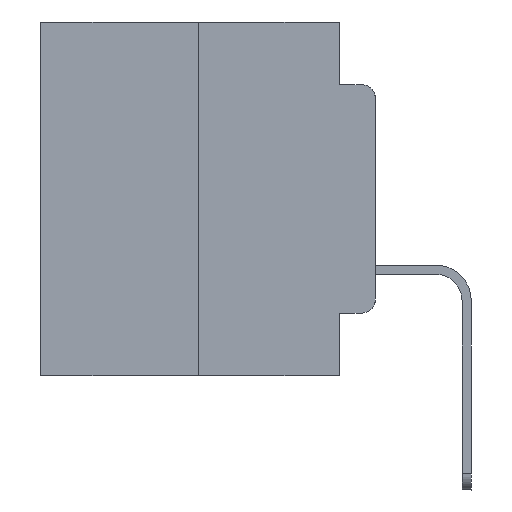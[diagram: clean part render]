
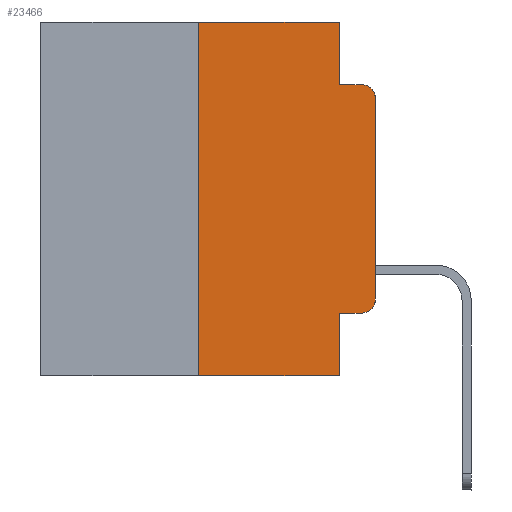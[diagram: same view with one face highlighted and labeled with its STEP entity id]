
A CAD part, left-side view. The second image highlights one B-rep face of the part: STEP entity #23466.
In plain terms, the highlighted planar face has unit normal (-1, 0, 0).
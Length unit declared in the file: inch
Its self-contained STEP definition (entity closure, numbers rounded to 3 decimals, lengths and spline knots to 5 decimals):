
#90 = EDGE_LOOP ( 'NONE', ( #7906, #20675, #12729, #15531, #20696, #12581, #9927, #1979, #15007, #8312 ) ) ;
#669 = VECTOR ( 'NONE', #8764, 39.37008 ) ;
#804 = LINE ( 'NONE', #24019, #14178 ) ;
#986 = LINE ( 'NONE', #20021, #14971 ) ;
#1452 = EDGE_CURVE ( 'NONE', #23525, #15380, #804, .T. ) ;
#1881 = LINE ( 'NONE', #20038, #669 ) ;
#1979 = ORIENTED_EDGE ( 'NONE', *, *, #7526, .F. ) ;
#1997 = VERTEX_POINT ( 'NONE', #24059 ) ;
#2972 = CARTESIAN_POINT ( 'NONE',  ( 0., 0., -0.3915 ) ) ;
#3052 = CARTESIAN_POINT ( 'NONE',  ( 0., 0.473, 0. ) ) ;
#3408 = FACE_OUTER_BOUND ( 'NONE', #90, .T. ) ;
#3547 = VECTOR ( 'NONE', #22465, 39.37008 ) ;
#4702 = DIRECTION ( 'NONE',  ( 0., -1., 0. ) ) ;
#4717 = EDGE_CURVE ( 'NONE', #17170, #5375, #19587, .T. ) ;
#4892 = LINE ( 'NONE', #21923, #9534 ) ;
#5129 = VERTEX_POINT ( 'NONE', #7682 ) ;
#5156 = DIRECTION ( 'NONE',  ( -1., 0., 0. ) ) ;
#5375 = VERTEX_POINT ( 'NONE', #7181 ) ;
#5620 = EDGE_CURVE ( 'NONE', #17170, #1997, #10167, .T. ) ;
#6285 = EDGE_CURVE ( 'NONE', #5375, #25774, #11062, .T. ) ;
#6389 = CARTESIAN_POINT ( 'NONE',  ( 0., 0.25, -0.5 ) ) ;
#7024 = VECTOR ( 'NONE', #4702, 39.37008 ) ;
#7181 = CARTESIAN_POINT ( 'NONE',  ( 0., 0.25, 0. ) ) ;
#7294 = CARTESIAN_POINT ( 'NONE',  ( 0., 0.02, -0.1085 ) ) ;
#7526 = EDGE_CURVE ( 'NONE', #5129, #1997, #25396, .T. ) ;
#7682 = CARTESIAN_POINT ( 'NONE',  ( 0., 0.051, -0.4115 ) ) ;
#7792 = VERTEX_POINT ( 'NONE', #15554 ) ;
#7906 = ORIENTED_EDGE ( 'NONE', *, *, #1452, .T. ) ;
#8046 = AXIS2_PLACEMENT_3D ( 'NONE', #3052, #10937, #24930 ) ;
#8052 = VECTOR ( 'NONE', #8599, 39.37008 ) ;
#8312 = ORIENTED_EDGE ( 'NONE', *, *, #14616, .T. ) ;
#8599 = DIRECTION ( 'NONE',  ( 0., 0., 1. ) ) ;
#8764 = DIRECTION ( 'NONE',  ( 0., 0., -1. ) ) ;
#9361 = VERTEX_POINT ( 'NONE', #19472 ) ;
#9534 = VECTOR ( 'NONE', #14000, 39.37008 ) ;
#9610 = CARTESIAN_POINT ( 'NONE',  ( 0., 0.473, -0.5 ) ) ;
#9927 = ORIENTED_EDGE ( 'NONE', *, *, #5620, .T. ) ;
#10167 = LINE ( 'NONE', #9610, #17958 ) ;
#10534 = CARTESIAN_POINT ( 'NONE',  ( 0., 0., -0.1085 ) ) ;
#10897 = CIRCLE ( 'NONE', #21399, 0.02 ) ;
#10937 = DIRECTION ( 'NONE',  ( 1., 0., 0. ) ) ;
#11062 = LINE ( 'NONE', #12573, #7024 ) ;
#11236 = AXIS2_PLACEMENT_3D ( 'NONE', #7294, #5156, #13043 ) ;
#12508 = CARTESIAN_POINT ( 'NONE',  ( 0., 0.25, 0. ) ) ;
#12573 = CARTESIAN_POINT ( 'NONE',  ( 0., 0.473, 0. ) ) ;
#12581 = ORIENTED_EDGE ( 'NONE', *, *, #4717, .F. ) ;
#12729 = ORIENTED_EDGE ( 'NONE', *, *, #22154, .F. ) ;
#13043 = DIRECTION ( 'NONE',  ( 0., 0., -1. ) ) ;
#13810 = DIRECTION ( 'NONE',  ( -1., 0., 0. ) ) ;
#14000 = DIRECTION ( 'NONE',  ( 0., -1., 0. ) ) ;
#14178 = VECTOR ( 'NONE', #14895, 39.37008 ) ;
#14616 = EDGE_CURVE ( 'NONE', #7792, #23525, #10897, .T. ) ;
#14816 = EDGE_CURVE ( 'NONE', #25774, #24749, #1881, .T. ) ;
#14895 = DIRECTION ( 'NONE',  ( 0., 0., 1. ) ) ;
#14971 = VECTOR ( 'NONE', #16196, 39.37008 ) ;
#15007 = ORIENTED_EDGE ( 'NONE', *, *, #25813, .T. ) ;
#15380 = VERTEX_POINT ( 'NONE', #10534 ) ;
#15531 = ORIENTED_EDGE ( 'NONE', *, *, #14816, .F. ) ;
#15554 = CARTESIAN_POINT ( 'NONE',  ( 0., 0.02, -0.4115 ) ) ;
#16012 = CARTESIAN_POINT ( 'NONE',  ( 0., 0.051, 0. ) ) ;
#16077 = EDGE_CURVE ( 'NONE', #15380, #9361, #23225, .T. ) ;
#16196 = DIRECTION ( 'NONE',  ( 0., -1., 0. ) ) ;
#17170 = VERTEX_POINT ( 'NONE', #6389 ) ;
#17626 = CARTESIAN_POINT ( 'NONE',  ( 0., 0.051, 0. ) ) ;
#17785 = DIRECTION ( 'NONE',  ( 0., 0., -1. ) ) ;
#17874 = CARTESIAN_POINT ( 'NONE',  ( 0., 0.02, -0.3915 ) ) ;
#17958 = VECTOR ( 'NONE', #23308, 39.37008 ) ;
#18569 = CARTESIAN_POINT ( 'NONE',  ( 0., 0.051, -0.0885 ) ) ;
#19472 = CARTESIAN_POINT ( 'NONE',  ( 0., 0.02, -0.0885 ) ) ;
#19587 = LINE ( 'NONE', #12508, #8052 ) ;
#20021 = CARTESIAN_POINT ( 'NONE',  ( 0., 0.051, -0.0885 ) ) ;
#20038 = CARTESIAN_POINT ( 'NONE',  ( 0., 0.051, 0. ) ) ;
#20614 = PLANE ( 'NONE',  #8046 ) ;
#20675 = ORIENTED_EDGE ( 'NONE', *, *, #16077, .T. ) ;
#20696 = ORIENTED_EDGE ( 'NONE', *, *, #6285, .F. ) ;
#21399 = AXIS2_PLACEMENT_3D ( 'NONE', #17874, #13810, #17785 ) ;
#21923 = CARTESIAN_POINT ( 'NONE',  ( 0., 0.051, -0.4115 ) ) ;
#22154 = EDGE_CURVE ( 'NONE', #24749, #9361, #986, .T. ) ;
#22465 = DIRECTION ( 'NONE',  ( 0., 0., -1. ) ) ;
#23225 = CIRCLE ( 'NONE', #11236, 0.02 ) ;
#23308 = DIRECTION ( 'NONE',  ( 0., -1., 0. ) ) ;
#23466 = ADVANCED_FACE ( 'NONE', ( #3408 ), #20614, .F. ) ;
#23525 = VERTEX_POINT ( 'NONE', #2972 ) ;
#24019 = CARTESIAN_POINT ( 'NONE',  ( 0., 0., 0. ) ) ;
#24059 = CARTESIAN_POINT ( 'NONE',  ( 0., 0.051, -0.5 ) ) ;
#24749 = VERTEX_POINT ( 'NONE', #18569 ) ;
#24930 = DIRECTION ( 'NONE',  ( 0., 0., -1. ) ) ;
#25396 = LINE ( 'NONE', #16012, #3547 ) ;
#25774 = VERTEX_POINT ( 'NONE', #17626 ) ;
#25813 = EDGE_CURVE ( 'NONE', #5129, #7792, #4892, .T. ) ;
